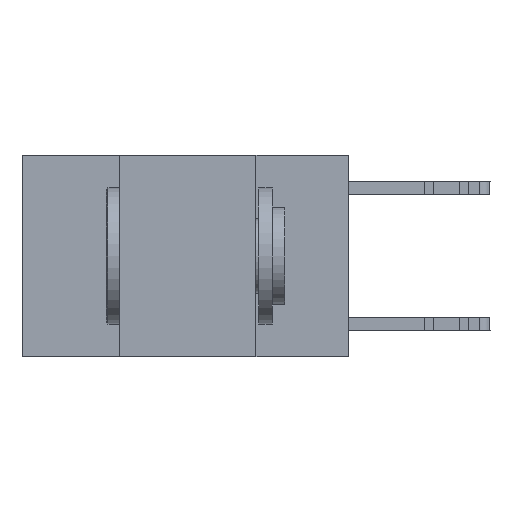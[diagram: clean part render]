
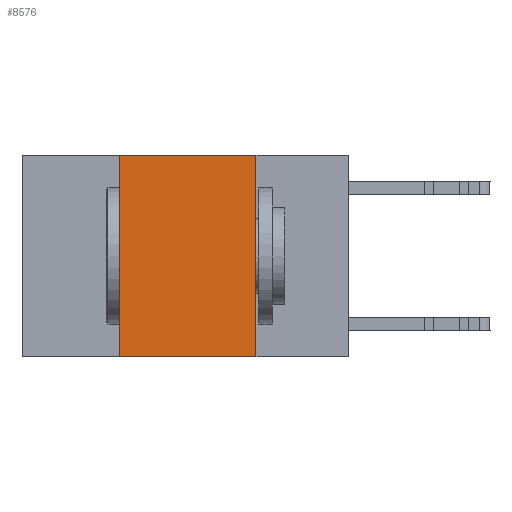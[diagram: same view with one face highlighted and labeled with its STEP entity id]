
A CAD part, left-side view. The second image highlights one B-rep face of the part: STEP entity #8576.
In plain terms, the highlighted planar face has unit normal (-1, 0, 0).
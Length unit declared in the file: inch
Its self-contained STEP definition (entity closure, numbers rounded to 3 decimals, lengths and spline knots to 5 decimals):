
#781 = CARTESIAN_POINT ( 'NONE',  ( 0., 0.17, 0. ) ) ;
#865 = DIRECTION ( 'NONE',  ( 0., -1., 0. ) ) ;
#1615 = EDGE_LOOP ( 'NONE', ( #21072, #26061, #22799, #6794 ) ) ;
#2331 = CARTESIAN_POINT ( 'NONE',  ( 0., 0.42, 0. ) ) ;
#3178 = DIRECTION ( 'NONE',  ( 0., 0., -1. ) ) ;
#3738 = DIRECTION ( 'NONE',  ( 0., 0., -1. ) ) ;
#4167 = CARTESIAN_POINT ( 'NONE',  ( 0., 0.17, 0. ) ) ;
#4187 = DIRECTION ( 'NONE',  ( 1., 0., 0. ) ) ;
#6688 = EDGE_CURVE ( 'NONE', #12893, #14500, #12329, .T. ) ;
#6794 = ORIENTED_EDGE ( 'NONE', *, *, #14170, .T. ) ;
#7206 = CARTESIAN_POINT ( 'NONE',  ( 0., 0.17, -0.37 ) ) ;
#8576 = ADVANCED_FACE ( 'NONE', ( #29682 ), #18369, .F. ) ;
#9554 = VECTOR ( 'NONE', #865, 39.37008 ) ;
#10185 = VERTEX_POINT ( 'NONE', #22887 ) ;
#12065 = VERTEX_POINT ( 'NONE', #29453 ) ;
#12329 = LINE ( 'NONE', #781, #23886 ) ;
#12425 = LINE ( 'NONE', #21748, #9554 ) ;
#12893 = VERTEX_POINT ( 'NONE', #4167 ) ;
#13168 = EDGE_CURVE ( 'NONE', #12065, #10185, #27814, .T. ) ;
#14033 = DIRECTION ( 'NONE',  ( 0., 0., 1. ) ) ;
#14170 = EDGE_CURVE ( 'NONE', #12065, #14500, #12425, .T. ) ;
#14500 = VERTEX_POINT ( 'NONE', #7206 ) ;
#14975 = CARTESIAN_POINT ( 'NONE',  ( 0., 0.6, 0. ) ) ;
#15527 = AXIS2_PLACEMENT_3D ( 'NONE', #25110, #4187, #3738 ) ;
#18369 = PLANE ( 'NONE',  #15527 ) ;
#18388 = EDGE_CURVE ( 'NONE', #10185, #12893, #26307, .T. ) ;
#18852 = VECTOR ( 'NONE', #14033, 39.37008 ) ;
#21072 = ORIENTED_EDGE ( 'NONE', *, *, #6688, .F. ) ;
#21748 = CARTESIAN_POINT ( 'NONE',  ( 0., 0.6, -0.37 ) ) ;
#22799 = ORIENTED_EDGE ( 'NONE', *, *, #13168, .F. ) ;
#22887 = CARTESIAN_POINT ( 'NONE',  ( 0., 0.42, 0. ) ) ;
#23886 = VECTOR ( 'NONE', #3178, 39.37008 ) ;
#25110 = CARTESIAN_POINT ( 'NONE',  ( 0., 0.6, 0. ) ) ;
#26061 = ORIENTED_EDGE ( 'NONE', *, *, #18388, .F. ) ;
#26307 = LINE ( 'NONE', #14975, #27552 ) ;
#27552 = VECTOR ( 'NONE', #28906, 39.37008 ) ;
#27814 = LINE ( 'NONE', #2331, #18852 ) ;
#28906 = DIRECTION ( 'NONE',  ( 0., -1., 0. ) ) ;
#29453 = CARTESIAN_POINT ( 'NONE',  ( 0., 0.42, -0.37 ) ) ;
#29682 = FACE_OUTER_BOUND ( 'NONE', #1615, .T. ) ;
